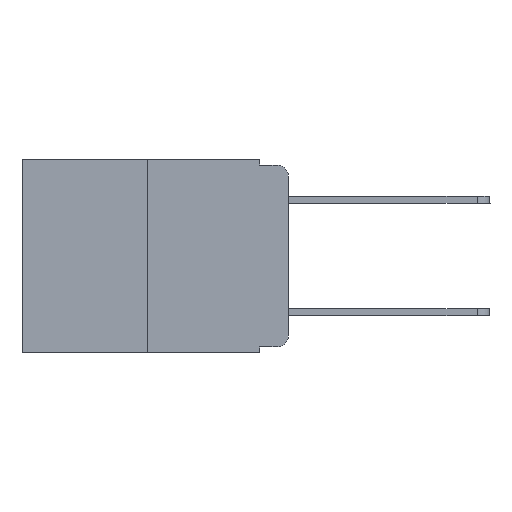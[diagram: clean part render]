
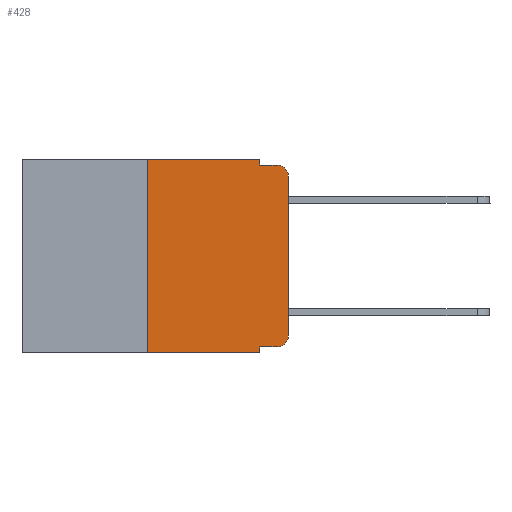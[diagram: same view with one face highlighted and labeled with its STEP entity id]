
A CAD part, left-side view. The second image highlights one B-rep face of the part: STEP entity #428.
In plain terms, the highlighted planar face has unit normal (-1, 0, 0).
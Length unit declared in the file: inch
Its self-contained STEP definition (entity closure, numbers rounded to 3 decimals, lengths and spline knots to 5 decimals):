
#428 = ADVANCED_FACE ( 'NONE', ( #6022 ), #21970, .F. ) ;
#543 = CIRCLE ( 'NONE', #26079, 0.02 ) ;
#859 = EDGE_CURVE ( 'NONE', #24015, #20606, #19278, .T. ) ;
#1276 = CARTESIAN_POINT ( 'NONE',  ( 0., 0.051, -0.01 ) ) ;
#2424 = ORIENTED_EDGE ( 'NONE', *, *, #859, .T. ) ;
#3788 = DIRECTION ( 'NONE',  ( 0., 0., -1. ) ) ;
#3931 = ORIENTED_EDGE ( 'NONE', *, *, #15628, .F. ) ;
#4011 = VECTOR ( 'NONE', #5893, 39.37008 ) ;
#4181 = LINE ( 'NONE', #1276, #19688 ) ;
#4387 = CARTESIAN_POINT ( 'NONE',  ( 0., 0.051, 0. ) ) ;
#5102 = ORIENTED_EDGE ( 'NONE', *, *, #21679, .F. ) ;
#5404 = EDGE_CURVE ( 'NONE', #15105, #24692, #4181, .T. ) ;
#5562 = AXIS2_PLACEMENT_3D ( 'NONE', #23998, #11876, #3788 ) ;
#5893 = DIRECTION ( 'NONE',  ( 0., 0., 1. ) ) ;
#6022 = FACE_OUTER_BOUND ( 'NONE', #24346, .T. ) ;
#6177 = DIRECTION ( 'NONE',  ( 0., 0., -1. ) ) ;
#6250 = LINE ( 'NONE', #21917, #4011 ) ;
#8045 = DIRECTION ( 'NONE',  ( 0., 0., -1. ) ) ;
#8525 = CARTESIAN_POINT ( 'NONE',  ( 0., 0., -0.313 ) ) ;
#8703 = VERTEX_POINT ( 'NONE', #23109 ) ;
#9055 = EDGE_CURVE ( 'NONE', #11721, #24692, #543, .T. ) ;
#9548 = VECTOR ( 'NONE', #15355, 39.37008 ) ;
#10319 = CARTESIAN_POINT ( 'NONE',  ( 0., 0.051, -0.333 ) ) ;
#10337 = ORIENTED_EDGE ( 'NONE', *, *, #18384, .T. ) ;
#10847 = AXIS2_PLACEMENT_3D ( 'NONE', #16242, #18182, #20394 ) ;
#10988 = CARTESIAN_POINT ( 'NONE',  ( 0., 0.02, -0.333 ) ) ;
#11620 = VECTOR ( 'NONE', #15308, 39.37008 ) ;
#11688 = LINE ( 'NONE', #17844, #23716 ) ;
#11721 = VERTEX_POINT ( 'NONE', #20243 ) ;
#11876 = DIRECTION ( 'NONE',  ( 1., 0., 0. ) ) ;
#12223 = ORIENTED_EDGE ( 'NONE', *, *, #9055, .T. ) ;
#12368 = CARTESIAN_POINT ( 'NONE',  ( 0., 0.051, 0. ) ) ;
#12388 = EDGE_CURVE ( 'NONE', #15823, #15105, #18454, .T. ) ;
#12770 = VERTEX_POINT ( 'NONE', #15423 ) ;
#13148 = ORIENTED_EDGE ( 'NONE', *, *, #12388, .F. ) ;
#13256 = EDGE_CURVE ( 'NONE', #16403, #24015, #24598, .T. ) ;
#13971 = LINE ( 'NONE', #25369, #9548 ) ;
#14232 = CARTESIAN_POINT ( 'NONE',  ( 0., 0.051, -0.01 ) ) ;
#14640 = VECTOR ( 'NONE', #18425, 39.37008 ) ;
#14992 = VECTOR ( 'NONE', #6177, 39.37008 ) ;
#15105 = VERTEX_POINT ( 'NONE', #14232 ) ;
#15308 = DIRECTION ( 'NONE',  ( 0., -1., 0. ) ) ;
#15335 = ORIENTED_EDGE ( 'NONE', *, *, #13256, .T. ) ;
#15355 = DIRECTION ( 'NONE',  ( 0., -1., 0. ) ) ;
#15423 = CARTESIAN_POINT ( 'NONE',  ( 0., 0.051, -0.343 ) ) ;
#15436 = CARTESIAN_POINT ( 'NONE',  ( 0., 0.25, 0. ) ) ;
#15628 = EDGE_CURVE ( 'NONE', #16403, #12770, #25468, .T. ) ;
#15823 = VERTEX_POINT ( 'NONE', #4387 ) ;
#16082 = CARTESIAN_POINT ( 'NONE',  ( 0., 0.051, 0. ) ) ;
#16242 = CARTESIAN_POINT ( 'NONE',  ( 0., 0.02, -0.313 ) ) ;
#16403 = VERTEX_POINT ( 'NONE', #10319 ) ;
#16425 = EDGE_CURVE ( 'NONE', #20606, #11721, #25417, .T. ) ;
#16869 = EDGE_CURVE ( 'NONE', #17025, #15823, #13971, .T. ) ;
#17025 = VERTEX_POINT ( 'NONE', #15436 ) ;
#17844 = CARTESIAN_POINT ( 'NONE',  ( 0., 0.473, -0.343 ) ) ;
#18182 = DIRECTION ( 'NONE',  ( -1., 0., 0. ) ) ;
#18384 = EDGE_CURVE ( 'NONE', #8703, #12770, #11688, .T. ) ;
#18425 = DIRECTION ( 'NONE',  ( 0., 0., 1. ) ) ;
#18454 = LINE ( 'NONE', #12368, #14992 ) ;
#18785 = VECTOR ( 'NONE', #8045, 39.37008 ) ;
#19278 = CIRCLE ( 'NONE', #10847, 0.02 ) ;
#19688 = VECTOR ( 'NONE', #21510, 39.37008 ) ;
#20144 = CARTESIAN_POINT ( 'NONE',  ( 0., 0.02, -0.03 ) ) ;
#20243 = CARTESIAN_POINT ( 'NONE',  ( 0., 0., -0.03 ) ) ;
#20319 = DIRECTION ( 'NONE',  ( 0., 0., -1. ) ) ;
#20394 = DIRECTION ( 'NONE',  ( 0., 0., -1. ) ) ;
#20471 = ORIENTED_EDGE ( 'NONE', *, *, #16869, .F. ) ;
#20606 = VERTEX_POINT ( 'NONE', #8525 ) ;
#21510 = DIRECTION ( 'NONE',  ( 0., -1., 0. ) ) ;
#21679 = EDGE_CURVE ( 'NONE', #8703, #17025, #6250, .T. ) ;
#21917 = CARTESIAN_POINT ( 'NONE',  ( 0., 0.25, 0. ) ) ;
#21970 = PLANE ( 'NONE',  #5562 ) ;
#22013 = ORIENTED_EDGE ( 'NONE', *, *, #16425, .T. ) ;
#22203 = DIRECTION ( 'NONE',  ( 0., -1., 0. ) ) ;
#23109 = CARTESIAN_POINT ( 'NONE',  ( 0., 0.25, -0.343 ) ) ;
#23168 = ORIENTED_EDGE ( 'NONE', *, *, #5404, .F. ) ;
#23293 = CARTESIAN_POINT ( 'NONE',  ( 0., 0.051, -0.333 ) ) ;
#23716 = VECTOR ( 'NONE', #22203, 39.37008 ) ;
#23998 = CARTESIAN_POINT ( 'NONE',  ( 0., 0.473, 0. ) ) ;
#24015 = VERTEX_POINT ( 'NONE', #10988 ) ;
#24052 = DIRECTION ( 'NONE',  ( -1., 0., 0. ) ) ;
#24281 = CARTESIAN_POINT ( 'NONE',  ( 0., 0., 0. ) ) ;
#24346 = EDGE_LOOP ( 'NONE', ( #22013, #12223, #23168, #13148, #20471, #5102, #10337, #3931, #15335, #2424 ) ) ;
#24598 = LINE ( 'NONE', #23293, #11620 ) ;
#24692 = VERTEX_POINT ( 'NONE', #25133 ) ;
#25133 = CARTESIAN_POINT ( 'NONE',  ( 0., 0.02, -0.01 ) ) ;
#25369 = CARTESIAN_POINT ( 'NONE',  ( 0., 0.473, 0. ) ) ;
#25417 = LINE ( 'NONE', #24281, #14640 ) ;
#25468 = LINE ( 'NONE', #16082, #18785 ) ;
#26079 = AXIS2_PLACEMENT_3D ( 'NONE', #20144, #24052, #20319 ) ;
